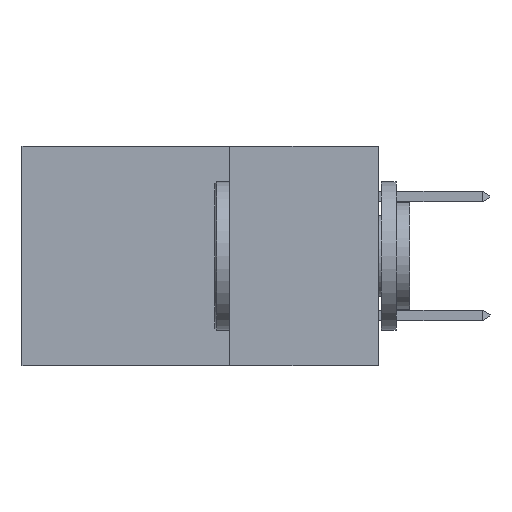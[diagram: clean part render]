
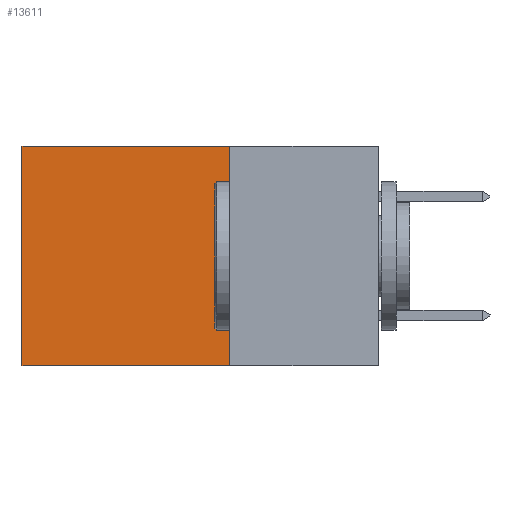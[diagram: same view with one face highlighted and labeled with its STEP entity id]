
A CAD part, left-side view. The second image highlights one B-rep face of the part: STEP entity #13611.
In plain terms, the highlighted planar face has unit normal (-1, 0, 0).
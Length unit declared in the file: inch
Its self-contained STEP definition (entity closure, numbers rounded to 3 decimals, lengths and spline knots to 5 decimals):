
#456 = VERTEX_POINT ( 'NONE', #13856 ) ;
#999 = EDGE_CURVE ( 'NONE', #9371, #12071, #10822, .T. ) ;
#1292 = AXIS2_PLACEMENT_3D ( 'NONE', #1326, #6615, #6612 ) ;
#1326 = CARTESIAN_POINT ( 'NONE',  ( 0.2615, 0.25, -0.37 ) ) ;
#2442 = EDGE_LOOP ( 'NONE', ( #15244, #12311, #14902, #12064 ) ) ;
#3183 = VECTOR ( 'NONE', #3848, 39.37008 ) ;
#3590 = CARTESIAN_POINT ( 'NONE',  ( 0.2615, 0.25, -0.37 ) ) ;
#3648 = PLANE ( 'NONE',  #1292 ) ;
#3777 = CARTESIAN_POINT ( 'NONE',  ( 0.2615, 0.25, 0. ) ) ;
#3848 = DIRECTION ( 'NONE',  ( 0., 1., 0. ) ) ;
#3886 = DIRECTION ( 'NONE',  ( 0., 1., 0. ) ) ;
#4497 = EDGE_CURVE ( 'NONE', #6349, #456, #13226, .T. ) ;
#5183 = VECTOR ( 'NONE', #15129, 39.37008 ) ;
#5893 = CARTESIAN_POINT ( 'NONE',  ( 0.2615, 0.25, 0. ) ) ;
#6349 = VERTEX_POINT ( 'NONE', #5893 ) ;
#6612 = DIRECTION ( 'NONE',  ( 0., 0., -1. ) ) ;
#6615 = DIRECTION ( 'NONE',  ( 1., 0., 0. ) ) ;
#7429 = VECTOR ( 'NONE', #3886, 39.37008 ) ;
#8015 = VECTOR ( 'NONE', #10674, 39.37008 ) ;
#8584 = LINE ( 'NONE', #15982, #5183 ) ;
#9371 = VERTEX_POINT ( 'NONE', #11680 ) ;
#9393 = FACE_OUTER_BOUND ( 'NONE', #2442, .T. ) ;
#9428 = EDGE_CURVE ( 'NONE', #6349, #9371, #11352, .T. ) ;
#10674 = DIRECTION ( 'NONE',  ( 0., 0., -1. ) ) ;
#10741 = CARTESIAN_POINT ( 'NONE',  ( 0.2615, 0.25, -0.37 ) ) ;
#10822 = LINE ( 'NONE', #3590, #7429 ) ;
#11352 = LINE ( 'NONE', #10741, #8015 ) ;
#11680 = CARTESIAN_POINT ( 'NONE',  ( 0.2615, 0.25, -0.37 ) ) ;
#12064 = ORIENTED_EDGE ( 'NONE', *, *, #4497, .T. ) ;
#12071 = VERTEX_POINT ( 'NONE', #15772 ) ;
#12311 = ORIENTED_EDGE ( 'NONE', *, *, #999, .F. ) ;
#13226 = LINE ( 'NONE', #3777, #3183 ) ;
#13611 = ADVANCED_FACE ( 'NONE', ( #9393 ), #3648, .F. ) ;
#13856 = CARTESIAN_POINT ( 'NONE',  ( 0.2615, 0.6, 0. ) ) ;
#14541 = EDGE_CURVE ( 'NONE', #456, #12071, #8584, .T. ) ;
#14902 = ORIENTED_EDGE ( 'NONE', *, *, #9428, .F. ) ;
#15129 = DIRECTION ( 'NONE',  ( 0., 0., -1. ) ) ;
#15244 = ORIENTED_EDGE ( 'NONE', *, *, #14541, .T. ) ;
#15772 = CARTESIAN_POINT ( 'NONE',  ( 0.2615, 0.6, -0.37 ) ) ;
#15982 = CARTESIAN_POINT ( 'NONE',  ( 0.2615, 0.6, -0.37 ) ) ;
